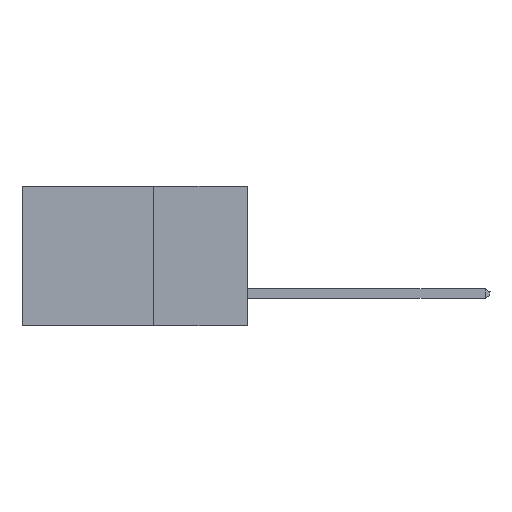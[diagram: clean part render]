
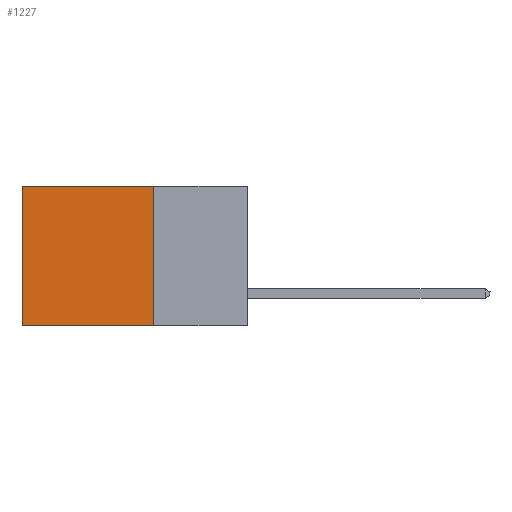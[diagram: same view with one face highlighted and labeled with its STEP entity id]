
A CAD part, left-side view. The second image highlights one B-rep face of the part: STEP entity #1227.
In plain terms, the highlighted planar face has unit normal (-1, 0, 0).
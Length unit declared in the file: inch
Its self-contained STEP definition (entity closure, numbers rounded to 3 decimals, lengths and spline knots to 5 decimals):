
#32 = LINE ( 'NONE', #3365, #2312 ) ;
#523 = CARTESIAN_POINT ( 'NONE',  ( 0.2615, 0.6, 0. ) ) ;
#528 = DIRECTION ( 'NONE',  ( 0., 1., 0. ) ) ;
#1104 = CARTESIAN_POINT ( 'NONE',  ( 0.2615, 0.6, -0.37 ) ) ;
#1175 = ORIENTED_EDGE ( 'NONE', *, *, #10457, .T. ) ;
#1227 = ADVANCED_FACE ( 'NONE', ( #3688 ), #3444, .F. ) ;
#1302 = ORIENTED_EDGE ( 'NONE', *, *, #6545, .F. ) ;
#1361 = LINE ( 'NONE', #6203, #1778 ) ;
#1368 = EDGE_CURVE ( 'NONE', #5545, #10029, #9712, .T. ) ;
#1778 = VECTOR ( 'NONE', #528, 39.37008 ) ;
#2041 = EDGE_LOOP ( 'NONE', ( #4414, #1302, #4876, #1175 ) ) ;
#2312 = VECTOR ( 'NONE', #6687, 39.37008 ) ;
#2878 = DIRECTION ( 'NONE',  ( 0., 0., -1. ) ) ;
#3028 = VECTOR ( 'NONE', #7048, 39.37008 ) ;
#3083 = VERTEX_POINT ( 'NONE', #523 ) ;
#3124 = VECTOR ( 'NONE', #3908, 39.37008 ) ;
#3365 = CARTESIAN_POINT ( 'NONE',  ( 0.2615, 0.6, -0.37 ) ) ;
#3444 = PLANE ( 'NONE',  #7598 ) ;
#3688 = FACE_OUTER_BOUND ( 'NONE', #2041, .T. ) ;
#3908 = DIRECTION ( 'NONE',  ( 0., 0., -1. ) ) ;
#4414 = ORIENTED_EDGE ( 'NONE', *, *, #7239, .T. ) ;
#4662 = CARTESIAN_POINT ( 'NONE',  ( 0.2615, 0.25, -0.37 ) ) ;
#4876 = ORIENTED_EDGE ( 'NONE', *, *, #1368, .F. ) ;
#5545 = VERTEX_POINT ( 'NONE', #7864 ) ;
#5860 = VERTEX_POINT ( 'NONE', #1104 ) ;
#6203 = CARTESIAN_POINT ( 'NONE',  ( 0.2615, 0.25, -0.37 ) ) ;
#6545 = EDGE_CURVE ( 'NONE', #10029, #5860, #1361, .T. ) ;
#6687 = DIRECTION ( 'NONE',  ( 0., 0., -1. ) ) ;
#7048 = DIRECTION ( 'NONE',  ( 0., 1., 0. ) ) ;
#7239 = EDGE_CURVE ( 'NONE', #3083, #5860, #32, .T. ) ;
#7598 = AXIS2_PLACEMENT_3D ( 'NONE', #9204, #9159, #2878 ) ;
#7864 = CARTESIAN_POINT ( 'NONE',  ( 0.2615, 0.25, 0. ) ) ;
#7917 = CARTESIAN_POINT ( 'NONE',  ( 0.2615, 0.25, 0. ) ) ;
#9159 = DIRECTION ( 'NONE',  ( 1., 0., 0. ) ) ;
#9204 = CARTESIAN_POINT ( 'NONE',  ( 0.2615, 0.25, -0.37 ) ) ;
#9712 = LINE ( 'NONE', #4662, #3124 ) ;
#10029 = VERTEX_POINT ( 'NONE', #10168 ) ;
#10168 = CARTESIAN_POINT ( 'NONE',  ( 0.2615, 0.25, -0.37 ) ) ;
#10299 = LINE ( 'NONE', #7917, #3028 ) ;
#10457 = EDGE_CURVE ( 'NONE', #5545, #3083, #10299, .T. ) ;
